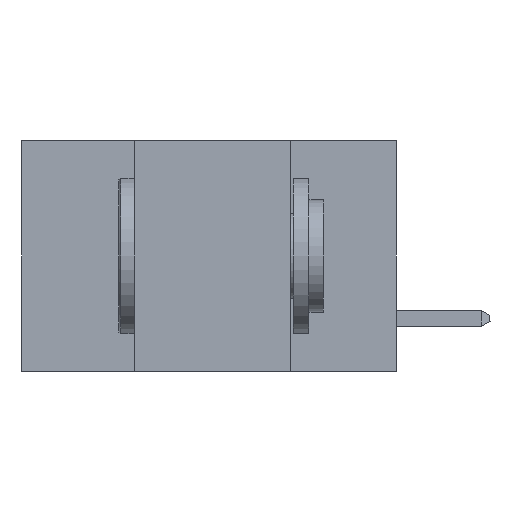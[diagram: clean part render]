
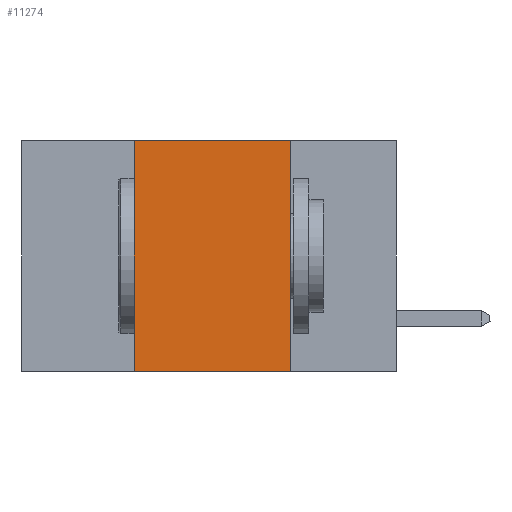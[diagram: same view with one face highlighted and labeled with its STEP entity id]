
A CAD part, left-side view. The second image highlights one B-rep face of the part: STEP entity #11274.
In plain terms, the highlighted planar face has unit normal (-1, 0, 0).
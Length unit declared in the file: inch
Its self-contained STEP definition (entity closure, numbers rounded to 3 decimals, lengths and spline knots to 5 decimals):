
#39 = ORIENTED_EDGE ( 'NONE', *, *, #12736, .F. ) ;
#205 = EDGE_LOOP ( 'NONE', ( #10932, #14070, #39, #4090 ) ) ;
#411 = LINE ( 'NONE', #6475, #7466 ) ;
#710 = DIRECTION ( 'NONE',  ( 0., -1., 0. ) ) ;
#1520 = EDGE_CURVE ( 'NONE', #6828, #7514, #411, .T. ) ;
#2158 = CARTESIAN_POINT ( 'NONE',  ( 0., 0.42, -0.37 ) ) ;
#3303 = VERTEX_POINT ( 'NONE', #12472 ) ;
#3548 = CARTESIAN_POINT ( 'NONE',  ( 0., 0.17, 0. ) ) ;
#3686 = DIRECTION ( 'NONE',  ( 0., 0., 1. ) ) ;
#4090 = ORIENTED_EDGE ( 'NONE', *, *, #8554, .T. ) ;
#4189 = CARTESIAN_POINT ( 'NONE',  ( 0., 0.42, 0. ) ) ;
#4544 = LINE ( 'NONE', #13888, #13562 ) ;
#4649 = CARTESIAN_POINT ( 'NONE',  ( 0., 0.6, 0. ) ) ;
#4771 = VECTOR ( 'NONE', #3686, 39.37008 ) ;
#5275 = EDGE_CURVE ( 'NONE', #7514, #3303, #9533, .T. ) ;
#5846 = PLANE ( 'NONE',  #10353 ) ;
#6475 = CARTESIAN_POINT ( 'NONE',  ( 0., 0.6, 0. ) ) ;
#6636 = VECTOR ( 'NONE', #8008, 39.37008 ) ;
#6828 = VERTEX_POINT ( 'NONE', #4189 ) ;
#6843 = CARTESIAN_POINT ( 'NONE',  ( 0., 0.17, -0.37 ) ) ;
#7460 = DIRECTION ( 'NONE',  ( 0., 0., -1. ) ) ;
#7466 = VECTOR ( 'NONE', #710, 39.37008 ) ;
#7514 = VERTEX_POINT ( 'NONE', #3548 ) ;
#7842 = LINE ( 'NONE', #11569, #4771 ) ;
#8008 = DIRECTION ( 'NONE',  ( 0., 0., -1. ) ) ;
#8224 = DIRECTION ( 'NONE',  ( 0., -1., 0. ) ) ;
#8554 = EDGE_CURVE ( 'NONE', #12547, #3303, #4544, .T. ) ;
#9533 = LINE ( 'NONE', #6843, #6636 ) ;
#10353 = AXIS2_PLACEMENT_3D ( 'NONE', #4649, #10515, #7460 ) ;
#10515 = DIRECTION ( 'NONE',  ( 1., 0., 0. ) ) ;
#10932 = ORIENTED_EDGE ( 'NONE', *, *, #5275, .F. ) ;
#11274 = ADVANCED_FACE ( 'NONE', ( #13479 ), #5846, .F. ) ;
#11569 = CARTESIAN_POINT ( 'NONE',  ( 0., 0.42, -0.37 ) ) ;
#12472 = CARTESIAN_POINT ( 'NONE',  ( 0., 0.17, -0.37 ) ) ;
#12547 = VERTEX_POINT ( 'NONE', #2158 ) ;
#12736 = EDGE_CURVE ( 'NONE', #12547, #6828, #7842, .T. ) ;
#13479 = FACE_OUTER_BOUND ( 'NONE', #205, .T. ) ;
#13562 = VECTOR ( 'NONE', #8224, 39.37008 ) ;
#13888 = CARTESIAN_POINT ( 'NONE',  ( 0., 0.6, -0.37 ) ) ;
#14070 = ORIENTED_EDGE ( 'NONE', *, *, #1520, .F. ) ;
